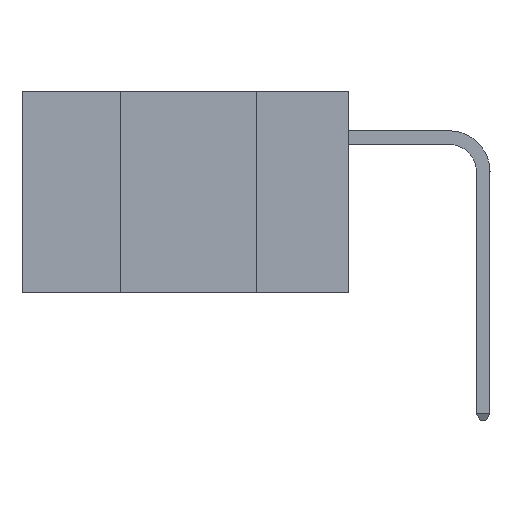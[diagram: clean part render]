
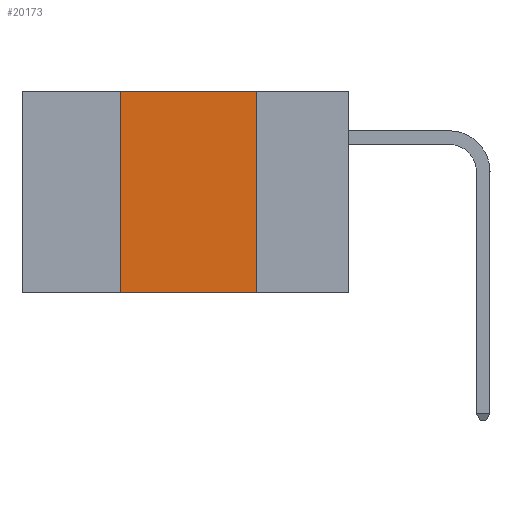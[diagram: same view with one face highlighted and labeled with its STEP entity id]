
A CAD part, left-side view. The second image highlights one B-rep face of the part: STEP entity #20173.
In plain terms, the highlighted planar face has unit normal (-1, 0, 0).
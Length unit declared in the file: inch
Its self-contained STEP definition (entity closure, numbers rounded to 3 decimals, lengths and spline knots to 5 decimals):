
#27 = DIRECTION ( 'NONE',  ( 0., 0., -1. ) ) ;
#5900 = AXIS2_PLACEMENT_3D ( 'NONE', #29626, #17843, #27 ) ;
#6000 = CARTESIAN_POINT ( 'NONE',  ( 0., 0.17, 0. ) ) ;
#10562 = ORIENTED_EDGE ( 'NONE', *, *, #24222, .F. ) ;
#10583 = EDGE_CURVE ( 'NONE', #31425, #13110, #36941, .T. ) ;
#11041 = CARTESIAN_POINT ( 'NONE',  ( 0., 0.17, -0.37 ) ) ;
#11159 = CARTESIAN_POINT ( 'NONE',  ( 0., 0.42, 0. ) ) ;
#12254 = EDGE_CURVE ( 'NONE', #24623, #13391, #30931, .T. ) ;
#13110 = VERTEX_POINT ( 'NONE', #33468 ) ;
#13385 = ORIENTED_EDGE ( 'NONE', *, *, #22229, .F. ) ;
#13391 = VERTEX_POINT ( 'NONE', #11041 ) ;
#13668 = VECTOR ( 'NONE', #30770, 39.37008 ) ;
#13857 = FACE_OUTER_BOUND ( 'NONE', #37588, .T. ) ;
#14041 = DIRECTION ( 'NONE',  ( 0., -1., 0. ) ) ;
#17843 = DIRECTION ( 'NONE',  ( 1., 0., 0. ) ) ;
#20173 = ADVANCED_FACE ( 'NONE', ( #13857 ), #35539, .F. ) ;
#20661 = CARTESIAN_POINT ( 'NONE',  ( 0., 0.6, -0.37 ) ) ;
#21296 = ORIENTED_EDGE ( 'NONE', *, *, #12254, .T. ) ;
#21389 = LINE ( 'NONE', #6000, #29241 ) ;
#21591 = LINE ( 'NONE', #30648, #13668 ) ;
#22229 = EDGE_CURVE ( 'NONE', #24623, #31425, #21591, .T. ) ;
#22565 = CARTESIAN_POINT ( 'NONE',  ( 0., 0.42, -0.37 ) ) ;
#24222 = EDGE_CURVE ( 'NONE', #13110, #13391, #21389, .T. ) ;
#24623 = VERTEX_POINT ( 'NONE', #22565 ) ;
#26374 = ORIENTED_EDGE ( 'NONE', *, *, #10583, .F. ) ;
#26592 = DIRECTION ( 'NONE',  ( 0., -1., 0. ) ) ;
#26728 = DIRECTION ( 'NONE',  ( 0., 0., -1. ) ) ;
#28194 = VECTOR ( 'NONE', #14041, 39.37008 ) ;
#29241 = VECTOR ( 'NONE', #26728, 39.37008 ) ;
#29626 = CARTESIAN_POINT ( 'NONE',  ( 0., 0.6, 0. ) ) ;
#30648 = CARTESIAN_POINT ( 'NONE',  ( 0., 0.42, 0. ) ) ;
#30770 = DIRECTION ( 'NONE',  ( 0., 0., 1. ) ) ;
#30931 = LINE ( 'NONE', #20661, #35986 ) ;
#31425 = VERTEX_POINT ( 'NONE', #11159 ) ;
#33468 = CARTESIAN_POINT ( 'NONE',  ( 0., 0.17, 0. ) ) ;
#34573 = CARTESIAN_POINT ( 'NONE',  ( 0., 0.6, 0. ) ) ;
#35539 = PLANE ( 'NONE',  #5900 ) ;
#35986 = VECTOR ( 'NONE', #26592, 39.37008 ) ;
#36941 = LINE ( 'NONE', #34573, #28194 ) ;
#37588 = EDGE_LOOP ( 'NONE', ( #10562, #26374, #13385, #21296 ) ) ;
